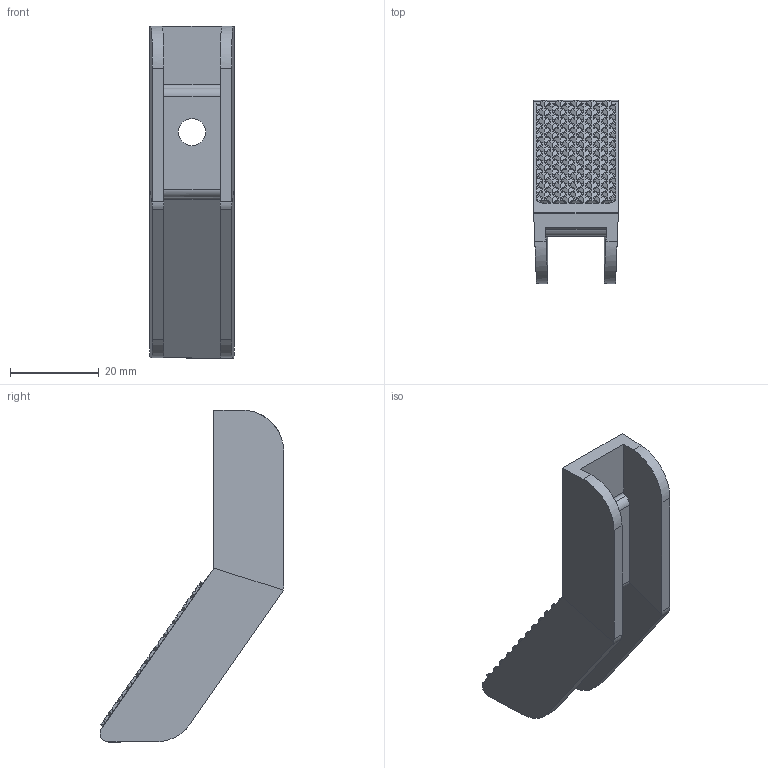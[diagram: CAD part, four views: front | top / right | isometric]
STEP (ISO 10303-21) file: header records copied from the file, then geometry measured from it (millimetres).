
FILE_DESCRIPTION (( 'STEP AP214' ), '1' );
FILE_NAME ('AR15-stock latch.STEP', '2013-06-18T15:27:49', ( 'Asher' ), ( '' ), 'SwSTEP 2.0', 'SolidWorks 2013', '' );
FILE_SCHEMA (( 'AUTOMOTIVE_DESIGN' ));
Length unit declared in the file: millimetre
Products named in the file (1): AR15-stock latch
Bounding box: 19.05 x 41.36 x 74.68 mm (x, y, z)
Volume: 10779.1 mm3; surface area: 8130.7 mm2
Topology: 1 solids, 1 shells, 640 faces, 1536 edges, 1024 vertices
Faces by surface type: plane 618, cylinder 22
Entity records: 18238 total; most frequent: CARTESIAN_POINT 3321, ORIENTED_EDGE 3072, DIRECTION 2798, EDGE_CURVE 1536, LINE 1476, VECTOR 1476, VERTEX_POINT 1024, EDGE_LOOP 768
